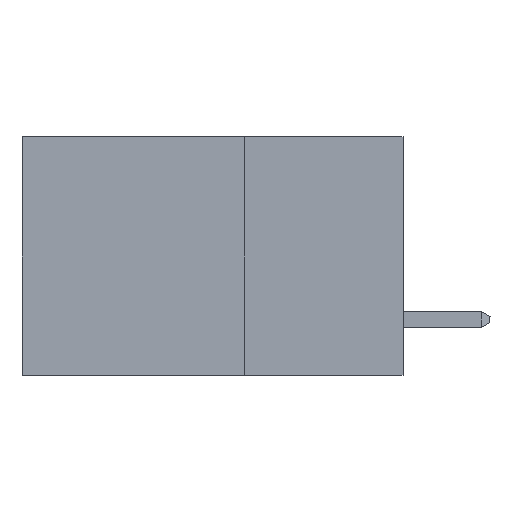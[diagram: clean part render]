
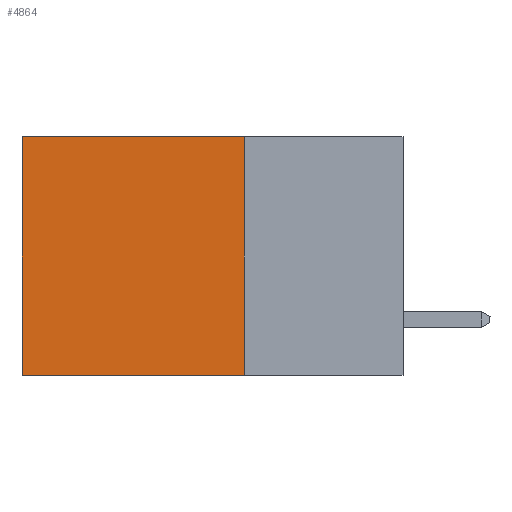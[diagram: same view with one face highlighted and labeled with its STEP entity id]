
A CAD part, left-side view. The second image highlights one B-rep face of the part: STEP entity #4864.
In plain terms, the highlighted planar face has unit normal (-1, 0, 0).
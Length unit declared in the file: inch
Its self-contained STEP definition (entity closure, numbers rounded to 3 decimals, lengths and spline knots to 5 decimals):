
#167 = ORIENTED_EDGE ( 'NONE', *, *, #4346, .T. ) ;
#1646 = EDGE_CURVE ( 'NONE', #15383, #12056, #3026, .T. ) ;
#1684 = LINE ( 'NONE', #9124, #4493 ) ;
#1742 = CARTESIAN_POINT ( 'NONE',  ( 0.2875, 0.6, -0.375 ) ) ;
#2245 = CARTESIAN_POINT ( 'NONE',  ( 0.2875, 0.25, -0.375 ) ) ;
#2309 = ORIENTED_EDGE ( 'NONE', *, *, #2569, .T. ) ;
#2569 = EDGE_CURVE ( 'NONE', #5365, #12056, #3836, .T. ) ;
#3026 = LINE ( 'NONE', #13687, #7782 ) ;
#3116 = EDGE_CURVE ( 'NONE', #8952, #15383, #6660, .T. ) ;
#3836 = LINE ( 'NONE', #1742, #11029 ) ;
#4346 = EDGE_CURVE ( 'NONE', #8952, #5365, #1684, .T. ) ;
#4493 = VECTOR ( 'NONE', #13698, 39.37008 ) ;
#4675 = EDGE_LOOP ( 'NONE', ( #2309, #7297, #9153, #167 ) ) ;
#4864 = ADVANCED_FACE ( 'NONE', ( #6437 ), #8974, .F. ) ;
#5365 = VERTEX_POINT ( 'NONE', #7381 ) ;
#6218 = VECTOR ( 'NONE', #11794, 39.37008 ) ;
#6437 = FACE_OUTER_BOUND ( 'NONE', #4675, .T. ) ;
#6660 = LINE ( 'NONE', #2245, #6218 ) ;
#7297 = ORIENTED_EDGE ( 'NONE', *, *, #1646, .F. ) ;
#7381 = CARTESIAN_POINT ( 'NONE',  ( 0.2875, 0.6, 0. ) ) ;
#7456 = DIRECTION ( 'NONE',  ( 1., 0., 0. ) ) ;
#7782 = VECTOR ( 'NONE', #12357, 39.37008 ) ;
#8952 = VERTEX_POINT ( 'NONE', #10728 ) ;
#8974 = PLANE ( 'NONE',  #12217 ) ;
#9124 = CARTESIAN_POINT ( 'NONE',  ( 0.2875, 0.25, 0. ) ) ;
#9153 = ORIENTED_EDGE ( 'NONE', *, *, #3116, .F. ) ;
#9317 = CARTESIAN_POINT ( 'NONE',  ( 0.2875, 0.6, -0.375 ) ) ;
#10096 = DIRECTION ( 'NONE',  ( 0., 0., -1. ) ) ;
#10728 = CARTESIAN_POINT ( 'NONE',  ( 0.2875, 0.25, 0. ) ) ;
#11029 = VECTOR ( 'NONE', #10096, 39.37008 ) ;
#11344 = CARTESIAN_POINT ( 'NONE',  ( 0.2875, 0.25, -0.375 ) ) ;
#11794 = DIRECTION ( 'NONE',  ( 0., 0., -1. ) ) ;
#12056 = VERTEX_POINT ( 'NONE', #9317 ) ;
#12217 = AXIS2_PLACEMENT_3D ( 'NONE', #14583, #7456, #17188 ) ;
#12357 = DIRECTION ( 'NONE',  ( 0., 1., 0. ) ) ;
#13687 = CARTESIAN_POINT ( 'NONE',  ( 0.2875, 0.25, -0.375 ) ) ;
#13698 = DIRECTION ( 'NONE',  ( 0., 1., 0. ) ) ;
#14583 = CARTESIAN_POINT ( 'NONE',  ( 0.2875, 0.25, -0.375 ) ) ;
#15383 = VERTEX_POINT ( 'NONE', #11344 ) ;
#17188 = DIRECTION ( 'NONE',  ( 0., 0., -1. ) ) ;
